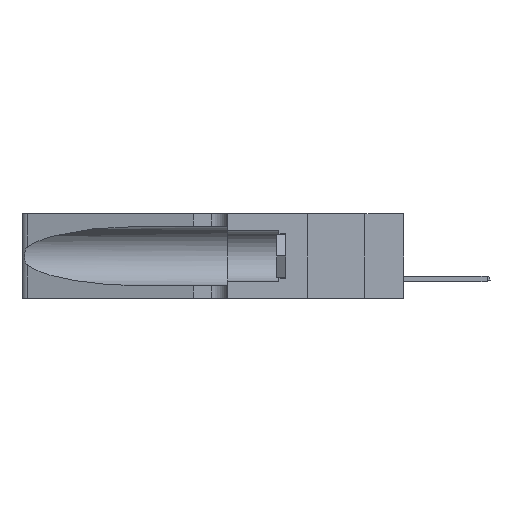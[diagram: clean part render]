
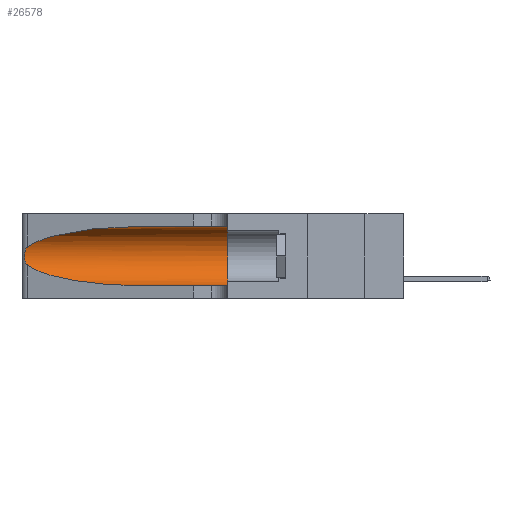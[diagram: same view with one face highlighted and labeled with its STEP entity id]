
A CAD part, left-side view. The second image highlights one B-rep face of the part: STEP entity #26578.
In plain terms, the highlighted cylindrical face has radius 3.308 mm (diameter 6.617 mm), a partial arc.
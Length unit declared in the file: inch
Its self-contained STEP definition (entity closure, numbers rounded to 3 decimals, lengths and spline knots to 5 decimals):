
#337 = CARTESIAN_POINT ( 'NONE',  ( 0.25787, 1.23484, 0.2124 ) ) ;
#360 = CARTESIAN_POINT ( 'NONE',  ( 0.1305, 0.35, 0.31525 ) ) ;
#1250 = CARTESIAN_POINT ( 'NONE',  ( 0.1305, 0.72297, 0.31525 ) ) ;
#1505 =( BOUNDED_CURVE ( )  B_SPLINE_CURVE ( 3, ( #35326, #20946, #3877, #4395 ),
 .UNSPECIFIED., .F., .F. ) 
 B_SPLINE_CURVE_WITH_KNOTS ( ( 4, 4 ),
 ( 1.5708, 2.84003 ),
 .UNSPECIFIED. ) 
 CURVE ( )  GEOMETRIC_REPRESENTATION_ITEM ( )  RATIONAL_B_SPLINE_CURVE ( ( 1., 0.87, 0.87, 1. ) ) 
 REPRESENTATION_ITEM ( '' )  );
#1918 = EDGE_CURVE ( 'NONE', #24997, #11754, #28927, .T. ) ;
#2357 = CARTESIAN_POINT ( 'NONE',  ( 0.25555, 1.22994, 0.2215 ) ) ;
#2975 = EDGE_LOOP ( 'NONE', ( #6965, #6059, #8470, #13501, #24442, #29738 ) ) ;
#3877 = CARTESIAN_POINT ( 'NONE',  ( 0.2373, 1.15595, 0.28018 ) ) ;
#3908 = CARTESIAN_POINT ( 'NONE',  ( 0.25854, 1.2359, 0.20912 ) ) ;
#4395 = CARTESIAN_POINT ( 'NONE',  ( 0.25487, 1.22718, 0.22369 ) ) ;
#4535 = DIRECTION ( 'NONE',  ( 0., -1., 0. ) ) ;
#6059 = ORIENTED_EDGE ( 'NONE', *, *, #1918, .T. ) ;
#6681 = CYLINDRICAL_SURFACE ( 'NONE', #26856, 0.13025 ) ;
#6965 = ORIENTED_EDGE ( 'NONE', *, *, #26104, .T. ) ;
#7534 = CARTESIAN_POINT ( 'NONE',  ( 0.1305, 1.61858, 0.31525 ) ) ;
#8136 = EDGE_CURVE ( 'NONE', #11754, #27266, #37005, .T. ) ;
#8470 = ORIENTED_EDGE ( 'NONE', *, *, #8136, .T. ) ;
#8741 = CARTESIAN_POINT ( 'NONE',  ( 0.25639, 1.23186, 0.15144 ) ) ;
#10374 = CARTESIAN_POINT ( 'NONE',  ( 0.1305, 0.72297, 0.05475 ) ) ;
#10440 = CARTESIAN_POINT ( 'NONE',  ( 0.25639, 1.23184, 0.21858 ) ) ;
#11754 = VERTEX_POINT ( 'NONE', #34624 ) ;
#11911 = CARTESIAN_POINT ( 'NONE',  ( 0.26075, 1.23896, 0.178 ) ) ;
#13081 = CIRCLE ( 'NONE', #25022, 0.13025 ) ;
#13424 = CARTESIAN_POINT ( 'NONE',  ( 0.18966, 0.96281, 0.05475 ) ) ;
#13501 = ORIENTED_EDGE ( 'NONE', *, *, #23836, .T. ) ;
#13793 = CARTESIAN_POINT ( 'NONE',  ( 0.1305, 0.72297, 0.05475 ) ) ;
#14013 = VECTOR ( 'NONE', #34825, 39.37008 ) ;
#14825 = CARTESIAN_POINT ( 'NONE',  ( 0.25789, 1.23486, 0.15765 ) ) ;
#15083 = CARTESIAN_POINT ( 'NONE',  ( 0.1305, 1.61858, 0.185 ) ) ;
#16083 = CARTESIAN_POINT ( 'NONE',  ( 0.26075, 1.23896, 0.19203 ) ) ;
#16557 = CARTESIAN_POINT ( 'NONE',  ( 0.25487, 1.22718, 0.14631 ) ) ;
#17147 = DIRECTION ( 'NONE',  ( 0., 0., 1. ) ) ;
#17773 = EDGE_CURVE ( 'NONE', #22410, #21274, #13081, .T. ) ;
#17834 = DIRECTION ( 'NONE',  ( 0., 0., -1. ) ) ;
#18251 = CARTESIAN_POINT ( 'NONE',  ( 0.1305, 0.35, 0.05475 ) ) ;
#19516 = CARTESIAN_POINT ( 'NONE',  ( 0.26018, 1.23835, 0.19895 ) ) ;
#20546 = CARTESIAN_POINT ( 'NONE',  ( 0.25487, 1.22718, 0.22369 ) ) ;
#20946 = CARTESIAN_POINT ( 'NONE',  ( 0.18966, 0.96281, 0.31525 ) ) ;
#21274 = VERTEX_POINT ( 'NONE', #18251 ) ;
#22371 = CARTESIAN_POINT ( 'NONE',  ( 0.25487, 1.22718, 0.22369 ) ) ;
#22410 = VERTEX_POINT ( 'NONE', #360 ) ;
#23168 = CARTESIAN_POINT ( 'NONE',  ( 0.25555, 1.22993, 0.14849 ) ) ;
#23836 = EDGE_CURVE ( 'NONE', #27266, #21274, #32765, .T. ) ;
#24442 = ORIENTED_EDGE ( 'NONE', *, *, #17773, .F. ) ;
#24997 = VERTEX_POINT ( 'NONE', #20546 ) ;
#25022 = AXIS2_PLACEMENT_3D ( 'NONE', #28378, #31412, #17147 ) ;
#25052 = CARTESIAN_POINT ( 'NONE',  ( 0.26017, 1.23833, 0.17102 ) ) ;
#25832 = VECTOR ( 'NONE', #4535, 39.37008 ) ;
#26104 = EDGE_CURVE ( 'NONE', #32417, #24997, #1505, .T. ) ;
#26186 = CARTESIAN_POINT ( 'NONE',  ( 0.1305, 1.61858, 0.05475 ) ) ;
#26524 = DIRECTION ( 'NONE',  ( 0., -1., 0. ) ) ;
#26578 = ADVANCED_FACE ( 'NONE', ( #30822 ), #6681, .F. ) ;
#26856 = AXIS2_PLACEMENT_3D ( 'NONE', #15083, #26524, #17834 ) ;
#27266 = VERTEX_POINT ( 'NONE', #10374 ) ;
#28378 = CARTESIAN_POINT ( 'NONE',  ( 0.1305, 0.35, 0.185 ) ) ;
#28521 = LINE ( 'NONE', #7534, #25832 ) ;
#28927 = B_SPLINE_CURVE_WITH_KNOTS ( 'NONE', 3,
 ( #22371, #2357, #10440, #337, #3908, #19516, #16083, #11911, #25052, #34545, #14825, #8741, #23168, #31580 ),
 .UNSPECIFIED., .F., .F.,
 ( 4, 2, 2, 2, 2, 2, 4 ),
 ( 0., 0.00027, 0.00053, 0.00107, 0.0016, 0.00187, 0.00214 ),
 .UNSPECIFIED. ) ;
#29738 = ORIENTED_EDGE ( 'NONE', *, *, #32469, .F. ) ;
#30822 = FACE_OUTER_BOUND ( 'NONE', #2975, .T. ) ;
#31412 = DIRECTION ( 'NONE',  ( 0., 1., 0. ) ) ;
#31580 = CARTESIAN_POINT ( 'NONE',  ( 0.25487, 1.22718, 0.14631 ) ) ;
#32417 = VERTEX_POINT ( 'NONE', #1250 ) ;
#32469 = EDGE_CURVE ( 'NONE', #32417, #22410, #28521, .T. ) ;
#32765 = LINE ( 'NONE', #26186, #14013 ) ;
#33658 = CARTESIAN_POINT ( 'NONE',  ( 0.2373, 1.15595, 0.08982 ) ) ;
#34545 = CARTESIAN_POINT ( 'NONE',  ( 0.25856, 1.23593, 0.16098 ) ) ;
#34624 = CARTESIAN_POINT ( 'NONE',  ( 0.25487, 1.22718, 0.14631 ) ) ;
#34825 = DIRECTION ( 'NONE',  ( 0., -1., 0. ) ) ;
#35326 = CARTESIAN_POINT ( 'NONE',  ( 0.1305, 0.72297, 0.31525 ) ) ;
#37005 =( BOUNDED_CURVE ( )  B_SPLINE_CURVE ( 3, ( #16557, #33658, #13424, #13793 ),
 .UNSPECIFIED., .F., .T. ) 
 B_SPLINE_CURVE_WITH_KNOTS ( ( 4, 4 ),
 ( 3.44316, 4.71239 ),
 .UNSPECIFIED. ) 
 CURVE ( )  GEOMETRIC_REPRESENTATION_ITEM ( )  RATIONAL_B_SPLINE_CURVE ( ( 1., 0.87, 0.87, 1. ) ) 
 REPRESENTATION_ITEM ( '' )  );
